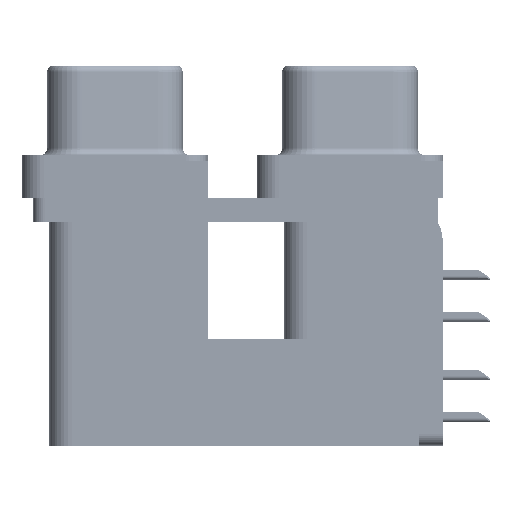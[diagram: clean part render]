
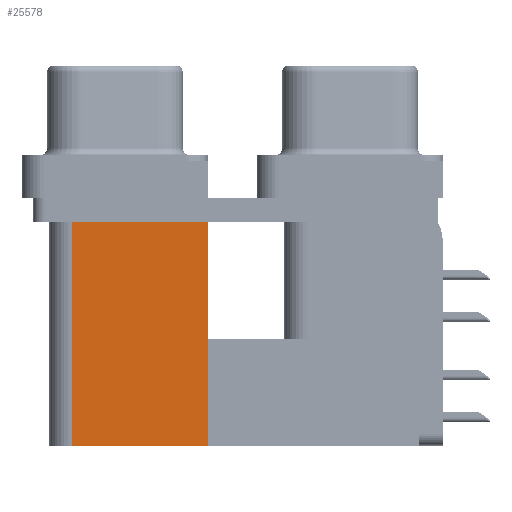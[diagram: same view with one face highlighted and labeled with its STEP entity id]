
A CAD part, left-side view. The second image highlights one B-rep face of the part: STEP entity #25578.
In plain terms, the highlighted planar face has unit normal (-1, 0, 0).
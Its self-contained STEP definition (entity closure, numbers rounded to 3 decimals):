
#1340 = DIRECTION ( 'NONE',  ( 0., 0., -1. ) ) ;
#2089 = DIRECTION ( 'NONE',  ( 1., 0., 0. ) ) ;
#3137 = VERTEX_POINT ( 'NONE', #29735 ) ;
#3421 = CARTESIAN_POINT ( 'NONE',  ( 3.79, 18.8, -19.2 ) ) ;
#3854 = LINE ( 'NONE', #6909, #10869 ) ;
#5714 = ORIENTED_EDGE ( 'NONE', *, *, #45742, .T. ) ;
#6909 = CARTESIAN_POINT ( 'NONE',  ( 3.79, 18.8, -19.2 ) ) ;
#7649 = EDGE_CURVE ( 'NONE', #40745, #46354, #27844, .T. ) ;
#8445 = VERTEX_POINT ( 'NONE', #44165 ) ;
#10869 = VECTOR ( 'NONE', #22568, 1000. ) ;
#11061 = CARTESIAN_POINT ( 'NONE',  ( 3.79, 9.6, -19.2 ) ) ;
#12887 = FACE_OUTER_BOUND ( 'NONE', #33750, .T. ) ;
#13112 = VECTOR ( 'NONE', #44860, 1000. ) ;
#13494 = LINE ( 'NONE', #29171, #13112 ) ;
#15558 = LINE ( 'NONE', #31221, #29878 ) ;
#17247 = CARTESIAN_POINT ( 'NONE',  ( 3.79, 9.6, -19.2 ) ) ;
#18961 = VECTOR ( 'NONE', #47150, 1000. ) ;
#20275 = ORIENTED_EDGE ( 'NONE', *, *, #7649, .F. ) ;
#22568 = DIRECTION ( 'NONE',  ( 0., 0., 1. ) ) ;
#23599 = ORIENTED_EDGE ( 'NONE', *, *, #50447, .T. ) ;
#25578 = ADVANCED_FACE ( 'NONE', ( #12887 ), #49110, .F. ) ;
#27844 = LINE ( 'NONE', #31446, #18961 ) ;
#29171 = CARTESIAN_POINT ( 'NONE',  ( 3.79, 9.6, -19.2 ) ) ;
#29735 = CARTESIAN_POINT ( 'NONE',  ( 3.79, 18.8, -2.5 ) ) ;
#29878 = VECTOR ( 'NONE', #46928, 1000. ) ;
#31221 = CARTESIAN_POINT ( 'NONE',  ( 3.79, 9.6, -2.5 ) ) ;
#31446 = CARTESIAN_POINT ( 'NONE',  ( 3.79, 9.6, -19.2 ) ) ;
#32502 = EDGE_CURVE ( 'NONE', #46354, #3137, #3854, .T. ) ;
#33750 = EDGE_LOOP ( 'NONE', ( #23599, #34610, #20275, #5714 ) ) ;
#34610 = ORIENTED_EDGE ( 'NONE', *, *, #32502, .F. ) ;
#40745 = VERTEX_POINT ( 'NONE', #11061 ) ;
#44165 = CARTESIAN_POINT ( 'NONE',  ( 3.79, 9.6, -2.5 ) ) ;
#44860 = DIRECTION ( 'NONE',  ( 0., 0., 1. ) ) ;
#45742 = EDGE_CURVE ( 'NONE', #40745, #8445, #13494, .T. ) ;
#46354 = VERTEX_POINT ( 'NONE', #3421 ) ;
#46928 = DIRECTION ( 'NONE',  ( 0., 1., 0. ) ) ;
#47150 = DIRECTION ( 'NONE',  ( 0., 1., 0. ) ) ;
#47280 = AXIS2_PLACEMENT_3D ( 'NONE', #17247, #2089, #1340 ) ;
#49110 = PLANE ( 'NONE',  #47280 ) ;
#50447 = EDGE_CURVE ( 'NONE', #8445, #3137, #15558, .T. ) ;
